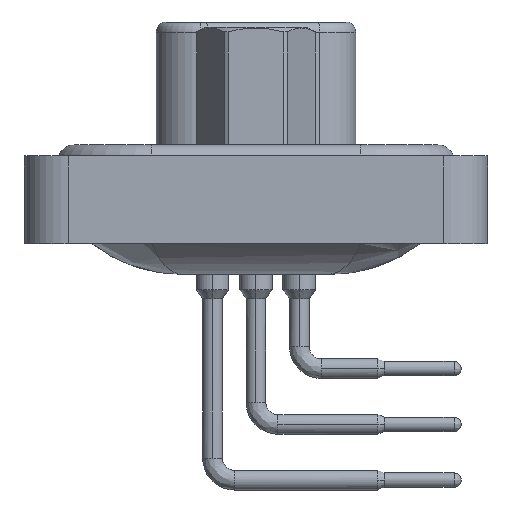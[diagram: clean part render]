
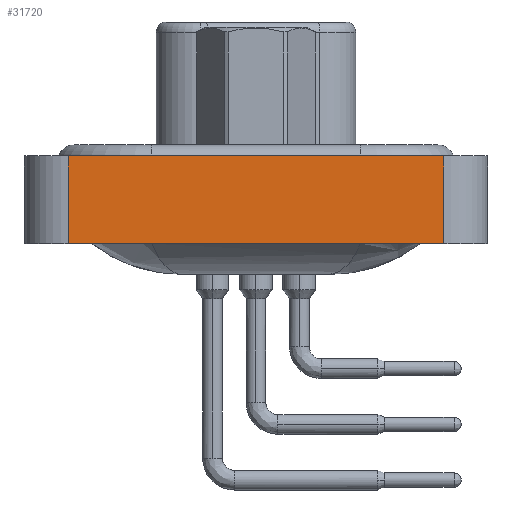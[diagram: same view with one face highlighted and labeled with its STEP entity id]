
A CAD part, left-side view. The second image highlights one B-rep face of the part: STEP entity #31720.
In plain terms, the highlighted planar face has unit normal (-1, 0, 0).
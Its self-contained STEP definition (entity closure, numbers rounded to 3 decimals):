
#1192 = CARTESIAN_POINT ( 'NONE',  ( -7.285, -8.55, -3.6 ) ) ;
#1564 = CARTESIAN_POINT ( 'NONE',  ( -7.285, 8.55, 0.4 ) ) ;
#3234 = DIRECTION ( 'NONE',  ( 0., -1., 0. ) ) ;
#3905 = ORIENTED_EDGE ( 'NONE', *, *, #34944, .F. ) ;
#4772 = VERTEX_POINT ( 'NONE', #21962 ) ;
#8177 = EDGE_LOOP ( 'NONE', ( #26852, #14662, #3905, #14260 ) ) ;
#8900 = DIRECTION ( 'NONE',  ( 0., 0., 1. ) ) ;
#10847 = VERTEX_POINT ( 'NONE', #32599 ) ;
#11000 = CARTESIAN_POINT ( 'NONE',  ( -7.285, -8.55, 0.4 ) ) ;
#11075 = VECTOR ( 'NONE', #13748, 1000. ) ;
#11468 = CARTESIAN_POINT ( 'NONE',  ( -7.285, -8.55, -3.6 ) ) ;
#11555 = PLANE ( 'NONE',  #22621 ) ;
#12721 = DIRECTION ( 'NONE',  ( 0., 0., 1. ) ) ;
#13748 = DIRECTION ( 'NONE',  ( 0., -1., 0. ) ) ;
#14260 = ORIENTED_EDGE ( 'NONE', *, *, #20913, .T. ) ;
#14662 = ORIENTED_EDGE ( 'NONE', *, *, #20765, .F. ) ;
#14952 = DIRECTION ( 'NONE',  ( 0., 0., 1. ) ) ;
#14964 = VECTOR ( 'NONE', #3234, 1000. ) ;
#16586 = LINE ( 'NONE', #1192, #22161 ) ;
#17102 = CARTESIAN_POINT ( 'NONE',  ( -7.285, -8.55, -3.6 ) ) ;
#18721 = VERTEX_POINT ( 'NONE', #32441 ) ;
#20396 = VERTEX_POINT ( 'NONE', #1564 ) ;
#20765 = EDGE_CURVE ( 'NONE', #20396, #4772, #33029, .T. ) ;
#20913 = EDGE_CURVE ( 'NONE', #18721, #10847, #29578, .T. ) ;
#21962 = CARTESIAN_POINT ( 'NONE',  ( -7.285, -8.55, 0.4 ) ) ;
#22161 = VECTOR ( 'NONE', #14952, 1000. ) ;
#22578 = EDGE_CURVE ( 'NONE', #10847, #4772, #16586, .T. ) ;
#22621 = AXIS2_PLACEMENT_3D ( 'NONE', #17102, #25363, #8900 ) ;
#24627 = LINE ( 'NONE', #26403, #31118 ) ;
#25363 = DIRECTION ( 'NONE',  ( -1., 0., 0. ) ) ;
#26403 = CARTESIAN_POINT ( 'NONE',  ( -7.285, 8.55, -3.6 ) ) ;
#26852 = ORIENTED_EDGE ( 'NONE', *, *, #22578, .T. ) ;
#29578 = LINE ( 'NONE', #11468, #14964 ) ;
#30968 = FACE_OUTER_BOUND ( 'NONE', #8177, .T. ) ;
#31118 = VECTOR ( 'NONE', #12721, 1000. ) ;
#31720 = ADVANCED_FACE ( 'NONE', ( #30968 ), #11555, .T. ) ;
#32441 = CARTESIAN_POINT ( 'NONE',  ( -7.285, 8.55, -3.6 ) ) ;
#32599 = CARTESIAN_POINT ( 'NONE',  ( -7.285, -8.55, -3.6 ) ) ;
#33029 = LINE ( 'NONE', #11000, #11075 ) ;
#34944 = EDGE_CURVE ( 'NONE', #18721, #20396, #24627, .T. ) ;
